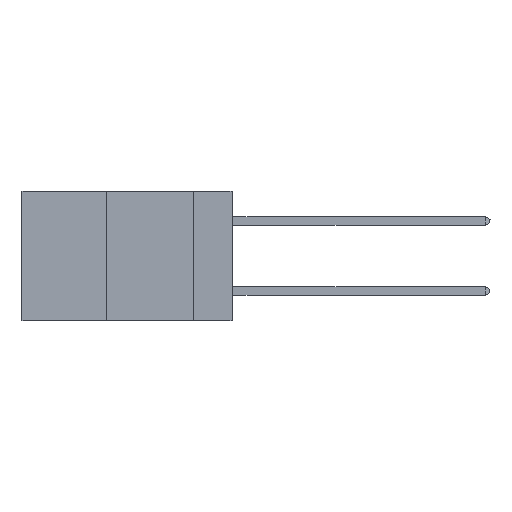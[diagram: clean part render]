
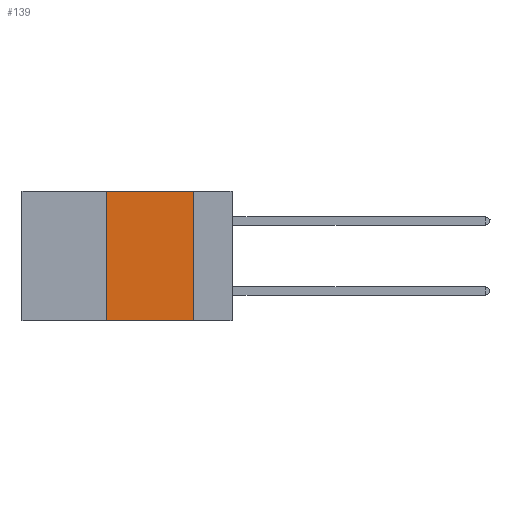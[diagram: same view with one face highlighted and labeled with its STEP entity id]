
A CAD part, left-side view. The second image highlights one B-rep face of the part: STEP entity #139.
In plain terms, the highlighted planar face has unit normal (-1, 0, 0).
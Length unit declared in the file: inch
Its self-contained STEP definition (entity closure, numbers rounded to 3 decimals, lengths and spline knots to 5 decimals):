
#72 = VERTEX_POINT ( 'NONE', #2489 ) ;
#139 = ADVANCED_FACE ( 'NONE', ( #23795 ), #7756, .F. ) ;
#1268 = ORIENTED_EDGE ( 'NONE', *, *, #10498, .T. ) ;
#2234 = EDGE_CURVE ( 'NONE', #4097, #20749, #4441, .T. ) ;
#2489 = CARTESIAN_POINT ( 'NONE',  ( 0., 0.11, -0.37 ) ) ;
#4097 = VERTEX_POINT ( 'NONE', #23232 ) ;
#4441 = LINE ( 'NONE', #20878, #7691 ) ;
#5724 = DIRECTION ( 'NONE',  ( 0., -1., 0. ) ) ;
#6500 = VECTOR ( 'NONE', #7903, 39.37008 ) ;
#6593 = DIRECTION ( 'NONE',  ( 0., -1., 0. ) ) ;
#7458 = EDGE_CURVE ( 'NONE', #20749, #13800, #11838, .T. ) ;
#7691 = VECTOR ( 'NONE', #12394, 39.37008 ) ;
#7756 = PLANE ( 'NONE',  #21933 ) ;
#7903 = DIRECTION ( 'NONE',  ( 0., 0., -1. ) ) ;
#9837 = CARTESIAN_POINT ( 'NONE',  ( 0., 0.36, 0. ) ) ;
#10498 = EDGE_CURVE ( 'NONE', #4097, #72, #16658, .T. ) ;
#10896 = EDGE_CURVE ( 'NONE', #13800, #72, #17960, .T. ) ;
#11143 = VECTOR ( 'NONE', #5724, 39.37008 ) ;
#11838 = LINE ( 'NONE', #19912, #11143 ) ;
#12394 = DIRECTION ( 'NONE',  ( 0., 0., 1. ) ) ;
#13800 = VERTEX_POINT ( 'NONE', #24184 ) ;
#15196 = DIRECTION ( 'NONE',  ( 0., 0., -1. ) ) ;
#16658 = LINE ( 'NONE', #16779, #21118 ) ;
#16779 = CARTESIAN_POINT ( 'NONE',  ( 0., 0.6, -0.37 ) ) ;
#17665 = CARTESIAN_POINT ( 'NONE',  ( 0., 0.6, 0. ) ) ;
#17866 = ORIENTED_EDGE ( 'NONE', *, *, #10896, .F. ) ;
#17879 = ORIENTED_EDGE ( 'NONE', *, *, #7458, .F. ) ;
#17960 = LINE ( 'NONE', #26076, #6500 ) ;
#18888 = ORIENTED_EDGE ( 'NONE', *, *, #2234, .F. ) ;
#19912 = CARTESIAN_POINT ( 'NONE',  ( 0., 0.6, 0. ) ) ;
#20270 = EDGE_LOOP ( 'NONE', ( #17866, #17879, #18888, #1268 ) ) ;
#20749 = VERTEX_POINT ( 'NONE', #9837 ) ;
#20878 = CARTESIAN_POINT ( 'NONE',  ( 0., 0.36, 0. ) ) ;
#21118 = VECTOR ( 'NONE', #6593, 39.37008 ) ;
#21933 = AXIS2_PLACEMENT_3D ( 'NONE', #17665, #22198, #15196 ) ;
#22198 = DIRECTION ( 'NONE',  ( 1., 0., 0. ) ) ;
#23232 = CARTESIAN_POINT ( 'NONE',  ( 0., 0.36, -0.37 ) ) ;
#23795 = FACE_OUTER_BOUND ( 'NONE', #20270, .T. ) ;
#24184 = CARTESIAN_POINT ( 'NONE',  ( 0., 0.11, 0. ) ) ;
#26076 = CARTESIAN_POINT ( 'NONE',  ( 0., 0.11, 0. ) ) ;
